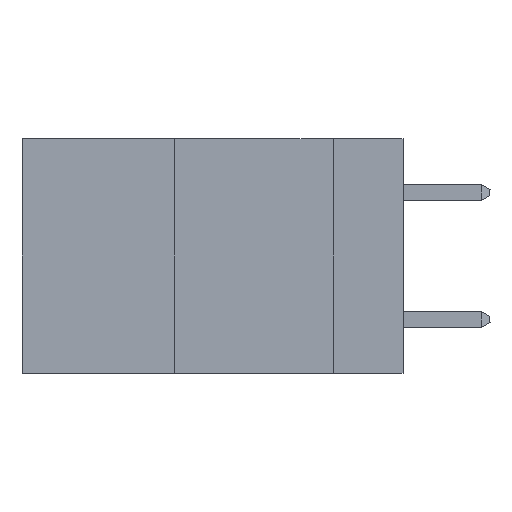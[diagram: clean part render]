
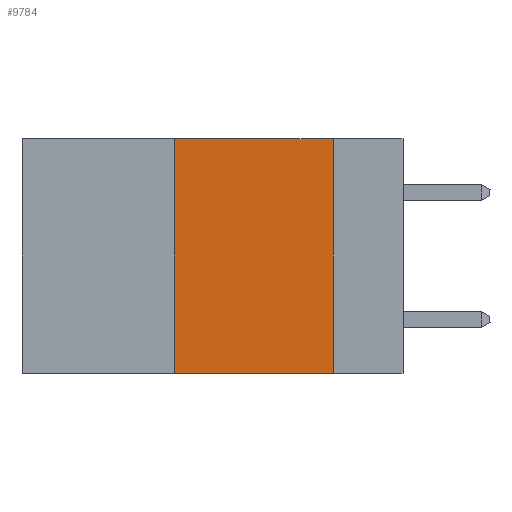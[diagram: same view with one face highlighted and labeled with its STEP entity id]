
A CAD part, left-side view. The second image highlights one B-rep face of the part: STEP entity #9784.
In plain terms, the highlighted planar face has unit normal (-1, 0, 0).
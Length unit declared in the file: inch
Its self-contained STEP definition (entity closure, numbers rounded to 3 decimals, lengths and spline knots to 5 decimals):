
#178 = LINE ( 'NONE', #13810, #12349 ) ;
#282 = ORIENTED_EDGE ( 'NONE', *, *, #1008, .F. ) ;
#750 = EDGE_CURVE ( 'NONE', #15113, #3627, #178, .T. ) ;
#1008 = EDGE_CURVE ( 'NONE', #15113, #2103, #5824, .T. ) ;
#1679 = VECTOR ( 'NONE', #12098, 39.37008 ) ;
#1875 = LINE ( 'NONE', #2223, #5250 ) ;
#1945 = DIRECTION ( 'NONE',  ( 0., 0., -1. ) ) ;
#2103 = VERTEX_POINT ( 'NONE', #17529 ) ;
#2115 = LINE ( 'NONE', #9218, #1679 ) ;
#2200 = VERTEX_POINT ( 'NONE', #4950 ) ;
#2223 = CARTESIAN_POINT ( 'NONE',  ( 0., 0.6, 0. ) ) ;
#2566 = ORIENTED_EDGE ( 'NONE', *, *, #4603, .F. ) ;
#3002 = CARTESIAN_POINT ( 'NONE',  ( 0., 0.36, -0.37 ) ) ;
#3627 = VERTEX_POINT ( 'NONE', #18617 ) ;
#3796 = VECTOR ( 'NONE', #12960, 39.37008 ) ;
#4092 = EDGE_CURVE ( 'NONE', #2200, #3627, #2115, .T. ) ;
#4603 = EDGE_CURVE ( 'NONE', #2103, #2200, #1875, .T. ) ;
#4950 = CARTESIAN_POINT ( 'NONE',  ( 0., 0.11, 0. ) ) ;
#5250 = VECTOR ( 'NONE', #10981, 39.37008 ) ;
#5824 = LINE ( 'NONE', #10025, #3796 ) ;
#6464 = CARTESIAN_POINT ( 'NONE',  ( 0., 0.6, 0. ) ) ;
#8509 = FACE_OUTER_BOUND ( 'NONE', #8559, .T. ) ;
#8559 = EDGE_LOOP ( 'NONE', ( #14008, #2566, #282, #11869 ) ) ;
#9218 = CARTESIAN_POINT ( 'NONE',  ( 0., 0.11, 0. ) ) ;
#9395 = DIRECTION ( 'NONE',  ( 1., 0., 0. ) ) ;
#9784 = ADVANCED_FACE ( 'NONE', ( #8509 ), #18479, .F. ) ;
#10025 = CARTESIAN_POINT ( 'NONE',  ( 0., 0.36, 0. ) ) ;
#10981 = DIRECTION ( 'NONE',  ( 0., -1., 0. ) ) ;
#11869 = ORIENTED_EDGE ( 'NONE', *, *, #750, .T. ) ;
#12098 = DIRECTION ( 'NONE',  ( 0., 0., -1. ) ) ;
#12334 = DIRECTION ( 'NONE',  ( 0., -1., 0. ) ) ;
#12349 = VECTOR ( 'NONE', #12334, 39.37008 ) ;
#12960 = DIRECTION ( 'NONE',  ( 0., 0., 1. ) ) ;
#13810 = CARTESIAN_POINT ( 'NONE',  ( 0., 0.6, -0.37 ) ) ;
#14008 = ORIENTED_EDGE ( 'NONE', *, *, #4092, .F. ) ;
#14900 = AXIS2_PLACEMENT_3D ( 'NONE', #6464, #9395, #1945 ) ;
#15113 = VERTEX_POINT ( 'NONE', #3002 ) ;
#17529 = CARTESIAN_POINT ( 'NONE',  ( 0., 0.36, 0. ) ) ;
#18479 = PLANE ( 'NONE',  #14900 ) ;
#18617 = CARTESIAN_POINT ( 'NONE',  ( 0., 0.11, -0.37 ) ) ;
